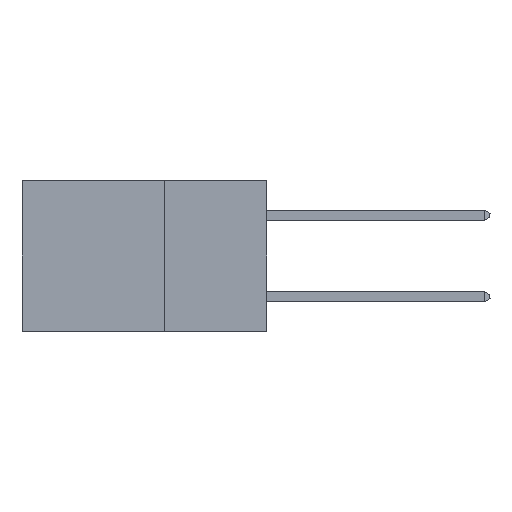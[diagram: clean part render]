
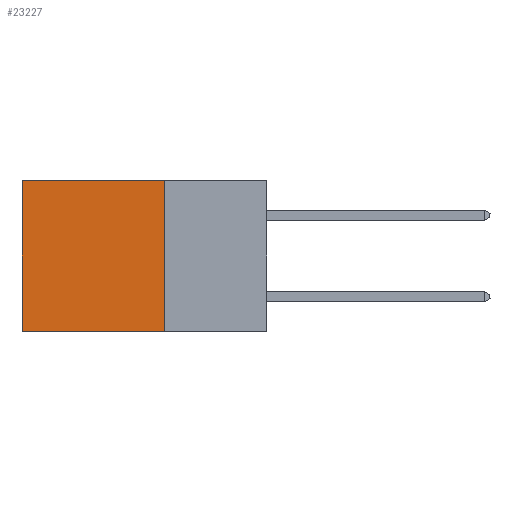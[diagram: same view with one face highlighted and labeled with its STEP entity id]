
A CAD part, left-side view. The second image highlights one B-rep face of the part: STEP entity #23227.
In plain terms, the highlighted planar face has unit normal (-1, 0, 0).
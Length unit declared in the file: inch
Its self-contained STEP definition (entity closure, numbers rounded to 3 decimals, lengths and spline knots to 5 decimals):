
#342 = LINE ( 'NONE', #26585, #26798 ) ;
#1248 = ORIENTED_EDGE ( 'NONE', *, *, #23913, .T. ) ;
#1273 = VECTOR ( 'NONE', #2745, 39.37008 ) ;
#1336 = LINE ( 'NONE', #23676, #17900 ) ;
#1803 = CARTESIAN_POINT ( 'NONE',  ( 0.2875, 0.25, 0. ) ) ;
#2745 = DIRECTION ( 'NONE',  ( 0., 0., -1. ) ) ;
#3501 = AXIS2_PLACEMENT_3D ( 'NONE', #16287, #16064, #7971 ) ;
#3952 = VERTEX_POINT ( 'NONE', #31266 ) ;
#6960 = CARTESIAN_POINT ( 'NONE',  ( 0.2875, 0.25, -0.37 ) ) ;
#7418 = EDGE_CURVE ( 'NONE', #3952, #13788, #19834, .T. ) ;
#7485 = LINE ( 'NONE', #28841, #1273 ) ;
#7971 = DIRECTION ( 'NONE',  ( 0., 0., -1. ) ) ;
#8245 = DIRECTION ( 'NONE',  ( 0., 1., 0. ) ) ;
#10732 = EDGE_CURVE ( 'NONE', #17221, #13788, #1336, .T. ) ;
#12474 = EDGE_CURVE ( 'NONE', #12911, #17221, #7485, .T. ) ;
#12911 = VERTEX_POINT ( 'NONE', #1803 ) ;
#13788 = VERTEX_POINT ( 'NONE', #18864 ) ;
#14965 = CARTESIAN_POINT ( 'NONE',  ( 0.2875, 0.6, 0. ) ) ;
#15138 = ORIENTED_EDGE ( 'NONE', *, *, #12474, .F. ) ;
#16064 = DIRECTION ( 'NONE',  ( 1., 0., 0. ) ) ;
#16287 = CARTESIAN_POINT ( 'NONE',  ( 0.2875, 0.25, 0. ) ) ;
#17009 = ORIENTED_EDGE ( 'NONE', *, *, #7418, .T. ) ;
#17221 = VERTEX_POINT ( 'NONE', #6960 ) ;
#17900 = VECTOR ( 'NONE', #34161, 39.37008 ) ;
#18864 = CARTESIAN_POINT ( 'NONE',  ( 0.2875, 0.6, -0.37 ) ) ;
#19834 = LINE ( 'NONE', #14965, #32997 ) ;
#20309 = DIRECTION ( 'NONE',  ( 0., 0., -1. ) ) ;
#22411 = FACE_OUTER_BOUND ( 'NONE', #29384, .T. ) ;
#23227 = ADVANCED_FACE ( 'NONE', ( #22411 ), #23787, .F. ) ;
#23676 = CARTESIAN_POINT ( 'NONE',  ( 0.2875, 0.25, -0.37 ) ) ;
#23787 = PLANE ( 'NONE',  #3501 ) ;
#23913 = EDGE_CURVE ( 'NONE', #12911, #3952, #342, .T. ) ;
#26585 = CARTESIAN_POINT ( 'NONE',  ( 0.2875, 0.25, 0. ) ) ;
#26798 = VECTOR ( 'NONE', #8245, 39.37008 ) ;
#28264 = ORIENTED_EDGE ( 'NONE', *, *, #10732, .F. ) ;
#28841 = CARTESIAN_POINT ( 'NONE',  ( 0.2875, 0.25, 0. ) ) ;
#29384 = EDGE_LOOP ( 'NONE', ( #17009, #28264, #15138, #1248 ) ) ;
#31266 = CARTESIAN_POINT ( 'NONE',  ( 0.2875, 0.6, 0. ) ) ;
#32997 = VECTOR ( 'NONE', #20309, 39.37008 ) ;
#34161 = DIRECTION ( 'NONE',  ( 0., 1., 0. ) ) ;
